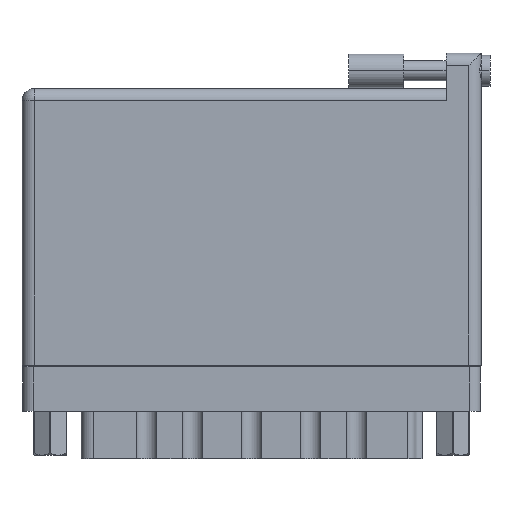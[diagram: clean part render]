
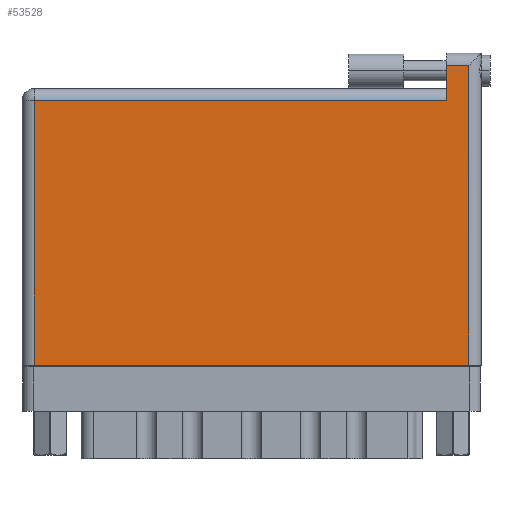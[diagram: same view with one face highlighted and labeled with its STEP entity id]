
A CAD part, front view. The second image highlights one B-rep face of the part: STEP entity #53528.
In plain terms, the highlighted face is planar.
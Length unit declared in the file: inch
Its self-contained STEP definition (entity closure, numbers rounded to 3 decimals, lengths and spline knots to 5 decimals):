
#3744 = CARTESIAN_POINT ( 'NONE',  ( 0., 0., 0. ) ) ;
#3834 = VECTOR ( 'NONE', #57418, 39.37008 ) ;
#4385 = LINE ( 'NONE', #24166, #44655 ) ;
#4455 = EDGE_CURVE ( 'NONE', #46789, #7949, #9076, .T. ) ;
#5985 = LINE ( 'NONE', #59076, #9876 ) ;
#6444 = AXIS2_PLACEMENT_3D ( 'NONE', #24872, #10435, #25180 ) ;
#7239 = ORIENTED_EDGE ( 'NONE', *, *, #33768, .T. ) ;
#7949 = VERTEX_POINT ( 'NONE', #20697 ) ;
#9076 = LINE ( 'NONE', #3744, #29871 ) ;
#9616 = DIRECTION ( 'NONE',  ( -1., 0., 0. ) ) ;
#9876 = VECTOR ( 'NONE', #25439, 39.37008 ) ;
#10435 = DIRECTION ( 'NONE',  ( 0., 0., -1. ) ) ;
#13189 = ORIENTED_EDGE ( 'NONE', *, *, #4455, .T. ) ;
#13383 = VERTEX_POINT ( 'NONE', #30529 ) ;
#19581 = EDGE_CURVE ( 'NONE', #46671, #13383, #37320, .T. ) ;
#20697 = CARTESIAN_POINT ( 'NONE',  ( 2.53, 0., 0. ) ) ;
#21135 = ORIENTED_EDGE ( 'NONE', *, *, #40614, .T. ) ;
#21578 = EDGE_CURVE ( 'NONE', #27849, #46789, #4385, .T. ) ;
#22892 = DIRECTION ( 'NONE',  ( 1., 0., 0. ) ) ;
#24061 = CARTESIAN_POINT ( 'NONE',  ( 0., 1.496, 0. ) ) ;
#24166 = CARTESIAN_POINT ( 'NONE',  ( 0.07, 0., 0. ) ) ;
#24872 = CARTESIAN_POINT ( 'NONE',  ( 0., 1.566, 0. ) ) ;
#25180 = DIRECTION ( 'NONE',  ( -1., 0., 0. ) ) ;
#25439 = DIRECTION ( 'NONE',  ( 0., 1., 0. ) ) ;
#26124 = FACE_OUTER_BOUND ( 'NONE', #48378, .T. ) ;
#27520 = LINE ( 'NONE', #24061, #33500 ) ;
#27849 = VERTEX_POINT ( 'NONE', #61966 ) ;
#29871 = VECTOR ( 'NONE', #22892, 39.37008 ) ;
#30529 = CARTESIAN_POINT ( 'NONE',  ( 2.403, 1.496, 0. ) ) ;
#32152 = CARTESIAN_POINT ( 'NONE',  ( 0.07, 0., 0. ) ) ;
#33500 = VECTOR ( 'NONE', #43241, 39.37008 ) ;
#33768 = EDGE_CURVE ( 'NONE', #13383, #27849, #27520, .T. ) ;
#37320 = LINE ( 'NONE', #56492, #3834 ) ;
#39336 = VECTOR ( 'NONE', #9616, 39.37008 ) ;
#39872 = ORIENTED_EDGE ( 'NONE', *, *, #21578, .T. ) ;
#40614 = EDGE_CURVE ( 'NONE', #7949, #43411, #5985, .T. ) ;
#42927 = CARTESIAN_POINT ( 'NONE',  ( 0., 1.696, 0. ) ) ;
#43241 = DIRECTION ( 'NONE',  ( -1., 0., 0. ) ) ;
#43411 = VERTEX_POINT ( 'NONE', #56288 ) ;
#44435 = ORIENTED_EDGE ( 'NONE', *, *, #19581, .T. ) ;
#44655 = VECTOR ( 'NONE', #47760, 39.37008 ) ;
#45299 = PLANE ( 'NONE',  #6444 ) ;
#46671 = VERTEX_POINT ( 'NONE', #60156 ) ;
#46789 = VERTEX_POINT ( 'NONE', #32152 ) ;
#47760 = DIRECTION ( 'NONE',  ( 0., -1., 0. ) ) ;
#48282 = LINE ( 'NONE', #42927, #39336 ) ;
#48378 = EDGE_LOOP ( 'NONE', ( #13189, #21135, #48954, #44435, #7239, #39872 ) ) ;
#48954 = ORIENTED_EDGE ( 'NONE', *, *, #51188, .T. ) ;
#51188 = EDGE_CURVE ( 'NONE', #43411, #46671, #48282, .T. ) ;
#53528 = ADVANCED_FACE ( 'NONE', ( #26124 ), #45299, .F. ) ;
#56288 = CARTESIAN_POINT ( 'NONE',  ( 2.53, 1.696, 0. ) ) ;
#56492 = CARTESIAN_POINT ( 'NONE',  ( 2.403, 1.766, 0. ) ) ;
#57418 = DIRECTION ( 'NONE',  ( 0., -1., 0. ) ) ;
#59076 = CARTESIAN_POINT ( 'NONE',  ( 2.53, 1.766, 0. ) ) ;
#60156 = CARTESIAN_POINT ( 'NONE',  ( 2.403, 1.696, 0. ) ) ;
#61966 = CARTESIAN_POINT ( 'NONE',  ( 0.07, 1.496, 0. ) ) ;
